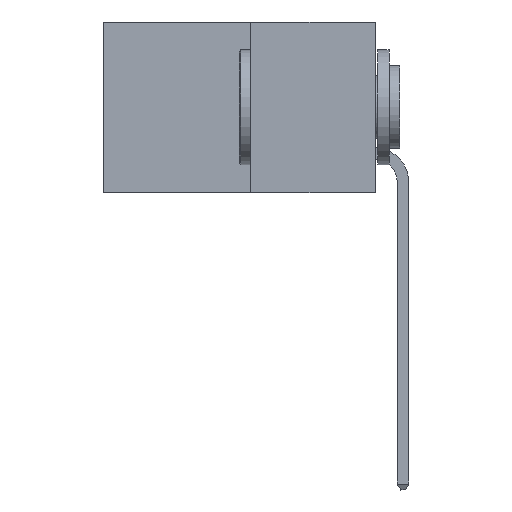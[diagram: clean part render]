
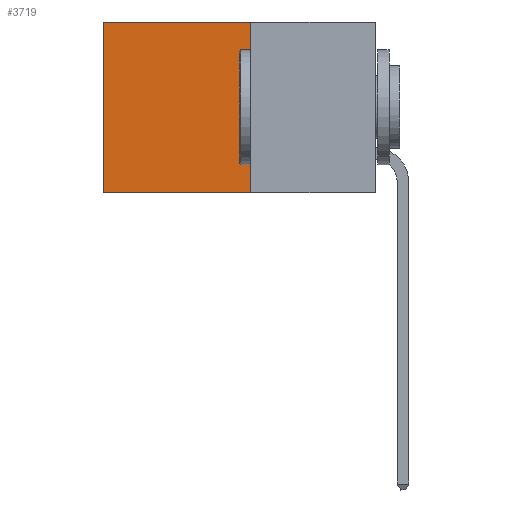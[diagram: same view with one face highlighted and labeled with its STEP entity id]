
A CAD part, left-side view. The second image highlights one B-rep face of the part: STEP entity #3719.
In plain terms, the highlighted planar face has unit normal (-1, 0, 0).
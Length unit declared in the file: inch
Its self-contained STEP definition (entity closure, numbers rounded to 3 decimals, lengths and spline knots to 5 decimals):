
#29 = DIRECTION ( 'NONE',  ( 0., 1., 0. ) ) ;
#52 = CARTESIAN_POINT ( 'NONE',  ( 0.277, 0.27, 0. ) ) ;
#53 = CARTESIAN_POINT ( 'NONE',  ( 0.277, 0.59, -0.37 ) ) ;
#2057 = DIRECTION ( 'NONE',  ( 0., 1., 0. ) ) ;
#2112 = LINE ( 'NONE', #5117, #11364 ) ;
#2496 = CARTESIAN_POINT ( 'NONE',  ( 0.277, 0.27, -0.37 ) ) ;
#3719 = ADVANCED_FACE ( 'NONE', ( #11291 ), #10127, .F. ) ;
#3805 = EDGE_CURVE ( 'NONE', #7040, #6794, #5908, .T. ) ;
#4595 = ORIENTED_EDGE ( 'NONE', *, *, #5629, .F. ) ;
#4642 = EDGE_LOOP ( 'NONE', ( #11284, #4595, #5911, #6431 ) ) ;
#4793 = DIRECTION ( 'NONE',  ( 0., 0., -1. ) ) ;
#5084 = VERTEX_POINT ( 'NONE', #7138 ) ;
#5117 = CARTESIAN_POINT ( 'NONE',  ( 0.277, 0.59, -0.37 ) ) ;
#5629 = EDGE_CURVE ( 'NONE', #6794, #8666, #9472, .T. ) ;
#5908 = LINE ( 'NONE', #8356, #8285 ) ;
#5911 = ORIENTED_EDGE ( 'NONE', *, *, #3805, .F. ) ;
#6135 = EDGE_CURVE ( 'NONE', #5084, #8666, #2112, .T. ) ;
#6431 = ORIENTED_EDGE ( 'NONE', *, *, #8672, .T. ) ;
#6794 = VERTEX_POINT ( 'NONE', #9869 ) ;
#7040 = VERTEX_POINT ( 'NONE', #8354 ) ;
#7063 = VECTOR ( 'NONE', #2057, 39.37008 ) ;
#7138 = CARTESIAN_POINT ( 'NONE',  ( 0.277, 0.59, 0. ) ) ;
#8285 = VECTOR ( 'NONE', #8321, 39.37008 ) ;
#8321 = DIRECTION ( 'NONE',  ( 0., 0., -1. ) ) ;
#8354 = CARTESIAN_POINT ( 'NONE',  ( 0.277, 0.27, 0. ) ) ;
#8356 = CARTESIAN_POINT ( 'NONE',  ( 0.277, 0.27, -0.37 ) ) ;
#8666 = VERTEX_POINT ( 'NONE', #53 ) ;
#8672 = EDGE_CURVE ( 'NONE', #7040, #5084, #11328, .T. ) ;
#9140 = VECTOR ( 'NONE', #29, 39.37008 ) ;
#9472 = LINE ( 'NONE', #2496, #7063 ) ;
#9869 = CARTESIAN_POINT ( 'NONE',  ( 0.277, 0.27, -0.37 ) ) ;
#10092 = DIRECTION ( 'NONE',  ( 0., 0., -1. ) ) ;
#10100 = DIRECTION ( 'NONE',  ( 1., 0., 0. ) ) ;
#10127 = PLANE ( 'NONE',  #11539 ) ;
#10135 = CARTESIAN_POINT ( 'NONE',  ( 0.277, 0.27, -0.37 ) ) ;
#11284 = ORIENTED_EDGE ( 'NONE', *, *, #6135, .T. ) ;
#11291 = FACE_OUTER_BOUND ( 'NONE', #4642, .T. ) ;
#11328 = LINE ( 'NONE', #52, #9140 ) ;
#11364 = VECTOR ( 'NONE', #4793, 39.37008 ) ;
#11539 = AXIS2_PLACEMENT_3D ( 'NONE', #10135, #10100, #10092 ) ;
